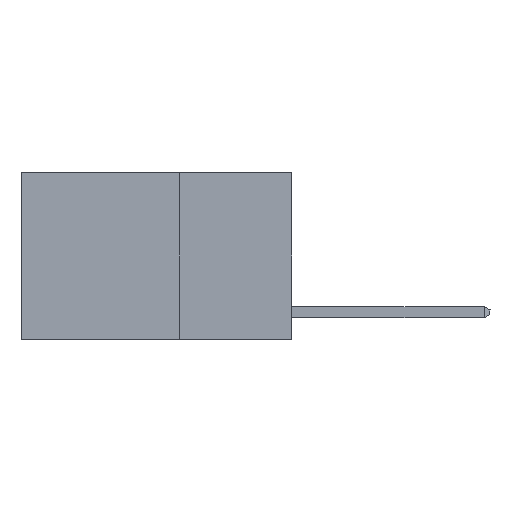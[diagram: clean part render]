
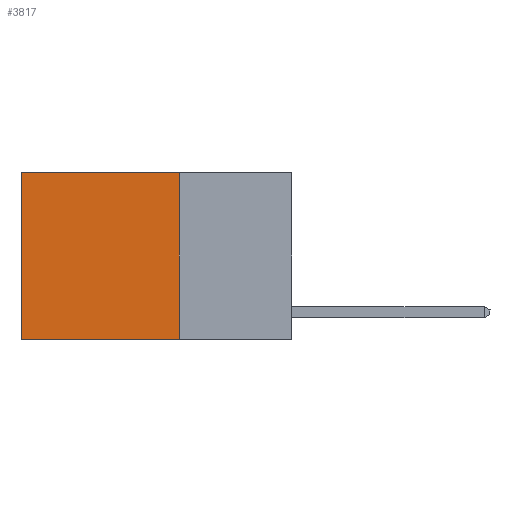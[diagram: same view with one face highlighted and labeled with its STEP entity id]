
A CAD part, left-side view. The second image highlights one B-rep face of the part: STEP entity #3817.
In plain terms, the highlighted planar face has unit normal (-1, 0, 0).
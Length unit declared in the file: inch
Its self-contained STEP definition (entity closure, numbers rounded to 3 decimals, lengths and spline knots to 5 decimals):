
#262 = VERTEX_POINT ( 'NONE', #10872 ) ;
#725 = CARTESIAN_POINT ( 'NONE',  ( 0.2625, 0.6, 0. ) ) ;
#798 = EDGE_LOOP ( 'NONE', ( #19934, #13128, #12823, #14460 ) ) ;
#1958 = LINE ( 'NONE', #17252, #21184 ) ;
#2544 = DIRECTION ( 'NONE',  ( 0., 0., -1. ) ) ;
#3255 = EDGE_CURVE ( 'NONE', #3879, #11373, #6144, .T. ) ;
#3817 = ADVANCED_FACE ( 'NONE', ( #12536 ), #8218, .F. ) ;
#3879 = VERTEX_POINT ( 'NONE', #8368 ) ;
#4288 = DIRECTION ( 'NONE',  ( 0., 1., 0. ) ) ;
#4481 = AXIS2_PLACEMENT_3D ( 'NONE', #21230, #23092, #11962 ) ;
#6054 = EDGE_CURVE ( 'NONE', #3879, #20775, #1958, .T. ) ;
#6144 = LINE ( 'NONE', #23205, #10546 ) ;
#6602 = DIRECTION ( 'NONE',  ( 0., 0., -1. ) ) ;
#7134 = LINE ( 'NONE', #8672, #11521 ) ;
#8218 = PLANE ( 'NONE',  #4481 ) ;
#8368 = CARTESIAN_POINT ( 'NONE',  ( 0.2625, 0.25, 0. ) ) ;
#8672 = CARTESIAN_POINT ( 'NONE',  ( 0.2625, 0.25, -0.37 ) ) ;
#10546 = VECTOR ( 'NONE', #6602, 39.37008 ) ;
#10872 = CARTESIAN_POINT ( 'NONE',  ( 0.2625, 0.6, -0.37 ) ) ;
#11373 = VERTEX_POINT ( 'NONE', #14591 ) ;
#11521 = VECTOR ( 'NONE', #19829, 39.37008 ) ;
#11638 = LINE ( 'NONE', #725, #15983 ) ;
#11962 = DIRECTION ( 'NONE',  ( 0., 0., -1. ) ) ;
#12536 = FACE_OUTER_BOUND ( 'NONE', #798, .T. ) ;
#12823 = ORIENTED_EDGE ( 'NONE', *, *, #3255, .F. ) ;
#13128 = ORIENTED_EDGE ( 'NONE', *, *, #19206, .F. ) ;
#14460 = ORIENTED_EDGE ( 'NONE', *, *, #6054, .T. ) ;
#14591 = CARTESIAN_POINT ( 'NONE',  ( 0.2625, 0.25, -0.37 ) ) ;
#15983 = VECTOR ( 'NONE', #2544, 39.37008 ) ;
#15996 = EDGE_CURVE ( 'NONE', #20775, #262, #11638, .T. ) ;
#17252 = CARTESIAN_POINT ( 'NONE',  ( 0.2625, 0.25, 0. ) ) ;
#18530 = CARTESIAN_POINT ( 'NONE',  ( 0.2625, 0.6, 0. ) ) ;
#19206 = EDGE_CURVE ( 'NONE', #11373, #262, #7134, .T. ) ;
#19829 = DIRECTION ( 'NONE',  ( 0., 1., 0. ) ) ;
#19934 = ORIENTED_EDGE ( 'NONE', *, *, #15996, .T. ) ;
#20775 = VERTEX_POINT ( 'NONE', #18530 ) ;
#21184 = VECTOR ( 'NONE', #4288, 39.37008 ) ;
#21230 = CARTESIAN_POINT ( 'NONE',  ( 0.2625, 0.25, 0. ) ) ;
#23092 = DIRECTION ( 'NONE',  ( 1., 0., 0. ) ) ;
#23205 = CARTESIAN_POINT ( 'NONE',  ( 0.2625, 0.25, 0. ) ) ;
